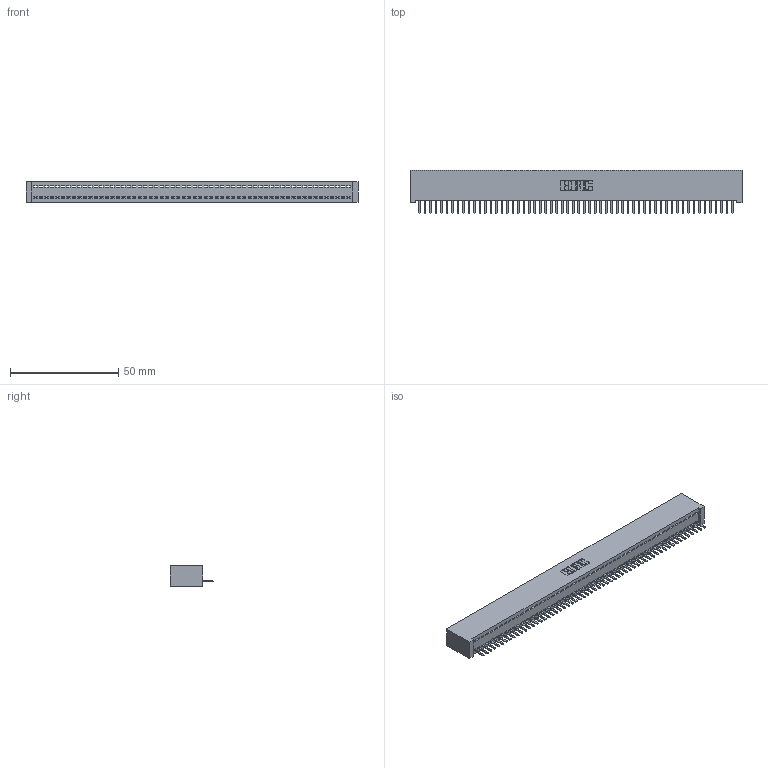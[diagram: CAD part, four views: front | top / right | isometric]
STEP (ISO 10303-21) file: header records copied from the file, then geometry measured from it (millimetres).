
FILE_DESCRIPTION (( 'STEP AP203' ), '1' );
FILE_NAME ('392-058-520-101.STEP', '2019-10-08T16:08:07', ( '' ), ( '' ), 'SwSTEP 2.0', 'SolidWorks 2016', '' );
FILE_SCHEMA (( 'CONFIG_CONTROL_DESIGN' ));
Length unit declared in the file: inch
Products named in the file (3): 342 Part_Lugless; 345-292-001_345-293-120; 392-058-520-101
Assembly tree (59 placements, depth 2):
  392-058-520-101
    342 Part_Lugless
    345-292-001_345-293-120  x58
Bounding box: 153.57 x 20.02 x 9.4 mm (x, y, z)
Volume: 13765.9 mm3; surface area: 20303.1 mm2
Topology: 59 solids, 59 shells, 3698 faces, 10947 edges, 7142 vertices
Faces by surface type: plane 2614, cylinder 1084
Entity records: 33093 total; most frequent: CARTESIAN_POINT 5724, ORIENTED_EDGE 5706, DIRECTION 4777, EDGE_CURVE 2853, VECTOR 2729, LINE 2729, VERTEX_POINT 1898, AXIS2_PLACEMENT_3D 1024
